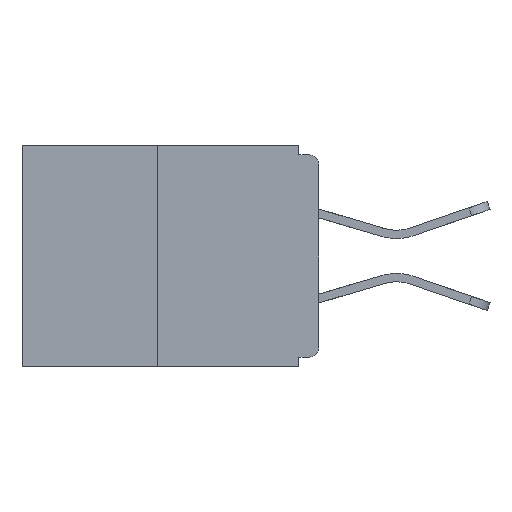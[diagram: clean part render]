
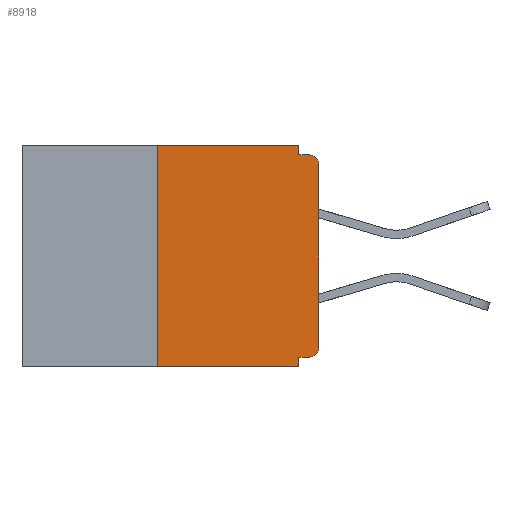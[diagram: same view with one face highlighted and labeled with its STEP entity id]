
A CAD part, left-side view. The second image highlights one B-rep face of the part: STEP entity #8918.
In plain terms, the highlighted planar face has unit normal (-1, 0, 0).
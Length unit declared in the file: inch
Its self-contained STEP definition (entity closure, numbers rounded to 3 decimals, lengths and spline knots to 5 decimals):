
#222 = EDGE_CURVE ( 'NONE', #14272, #4754, #8200, .T. ) ;
#387 = EDGE_CURVE ( 'NONE', #5098, #11218, #9555, .T. ) ;
#710 = DIRECTION ( 'NONE',  ( 0., -1., 0. ) ) ;
#914 = ORIENTED_EDGE ( 'NONE', *, *, #5044, .F. ) ;
#1134 = DIRECTION ( 'NONE',  ( 0., 0., -1. ) ) ;
#1265 = CARTESIAN_POINT ( 'NONE',  ( 0., 0.031, -0.015 ) ) ;
#1563 = CARTESIAN_POINT ( 'NONE',  ( 0., 0.031, -0.343 ) ) ;
#1713 = AXIS2_PLACEMENT_3D ( 'NONE', #7952, #4565, #1134 ) ;
#2033 = DIRECTION ( 'NONE',  ( 0., 0., -1. ) ) ;
#2289 = CARTESIAN_POINT ( 'NONE',  ( 0., 0.031, 0. ) ) ;
#2318 = ORIENTED_EDGE ( 'NONE', *, *, #8155, .F. ) ;
#2356 = AXIS2_PLACEMENT_3D ( 'NONE', #11083, #9074, #4626 ) ;
#2574 = CARTESIAN_POINT ( 'NONE',  ( 0., 0., -0.328 ) ) ;
#2588 = DIRECTION ( 'NONE',  ( 0., -1., 0. ) ) ;
#2750 = CARTESIAN_POINT ( 'NONE',  ( 0., 0.015, -0.313 ) ) ;
#2948 = VECTOR ( 'NONE', #13698, 39.37008 ) ;
#3143 = ORIENTED_EDGE ( 'NONE', *, *, #222, .T. ) ;
#3198 = EDGE_CURVE ( 'NONE', #12517, #14272, #5680, .T. ) ;
#3227 = VECTOR ( 'NONE', #10067, 39.37008 ) ;
#3420 = PLANE ( 'NONE',  #2356 ) ;
#3694 = EDGE_CURVE ( 'NONE', #13198, #4724, #12102, .T. ) ;
#3704 = CARTESIAN_POINT ( 'NONE',  ( 0., 0.015, -0.328 ) ) ;
#3873 = ORIENTED_EDGE ( 'NONE', *, *, #5990, .F. ) ;
#4414 = CARTESIAN_POINT ( 'NONE',  ( 0., 0.031, -0.343 ) ) ;
#4565 = DIRECTION ( 'NONE',  ( -1., 0., 0. ) ) ;
#4626 = DIRECTION ( 'NONE',  ( 0., 0., -1. ) ) ;
#4690 = ORIENTED_EDGE ( 'NONE', *, *, #10734, .T. ) ;
#4724 = VERTEX_POINT ( 'NONE', #1265 ) ;
#4754 = VERTEX_POINT ( 'NONE', #7933 ) ;
#5044 = EDGE_CURVE ( 'NONE', #11021, #13198, #8263, .T. ) ;
#5072 = VECTOR ( 'NONE', #11214, 39.37008 ) ;
#5098 = VERTEX_POINT ( 'NONE', #3704 ) ;
#5106 = VECTOR ( 'NONE', #2588, 39.37008 ) ;
#5109 = CARTESIAN_POINT ( 'NONE',  ( 0., 0., 0. ) ) ;
#5236 = CARTESIAN_POINT ( 'NONE',  ( 0., 0.25, 0. ) ) ;
#5571 = CARTESIAN_POINT ( 'NONE',  ( 0., 0., -0.313 ) ) ;
#5680 = LINE ( 'NONE', #5109, #7079 ) ;
#5990 = EDGE_CURVE ( 'NONE', #11218, #10954, #11665, .T. ) ;
#6112 = LINE ( 'NONE', #9053, #5072 ) ;
#6253 = CARTESIAN_POINT ( 'NONE',  ( 0., 0., -0.015 ) ) ;
#6674 = CARTESIAN_POINT ( 'NONE',  ( 0., 0.031, -0.328 ) ) ;
#6723 = ORIENTED_EDGE ( 'NONE', *, *, #13807, .F. ) ;
#6762 = CARTESIAN_POINT ( 'NONE',  ( 0., 0., -0.03 ) ) ;
#6983 = VECTOR ( 'NONE', #2033, 39.37008 ) ;
#7079 = VECTOR ( 'NONE', #9432, 39.37008 ) ;
#7489 = ORIENTED_EDGE ( 'NONE', *, *, #3198, .T. ) ;
#7549 = VERTEX_POINT ( 'NONE', #7600 ) ;
#7600 = CARTESIAN_POINT ( 'NONE',  ( 0., 0.25, -0.343 ) ) ;
#7933 = CARTESIAN_POINT ( 'NONE',  ( 0., 0.015, -0.015 ) ) ;
#7952 = CARTESIAN_POINT ( 'NONE',  ( 0., 0.015, -0.03 ) ) ;
#8155 = EDGE_CURVE ( 'NONE', #7549, #11021, #6112, .T. ) ;
#8200 = CIRCLE ( 'NONE', #1713, 0.015 ) ;
#8263 = LINE ( 'NONE', #11617, #5106 ) ;
#8517 = CIRCLE ( 'NONE', #13754, 0.015 ) ;
#8918 = ADVANCED_FACE ( 'NONE', ( #12882 ), #3420, .F. ) ;
#9046 = EDGE_CURVE ( 'NONE', #7549, #10954, #12865, .T. ) ;
#9053 = CARTESIAN_POINT ( 'NONE',  ( 0., 0.25, 0. ) ) ;
#9074 = DIRECTION ( 'NONE',  ( 1., 0., 0. ) ) ;
#9118 = CARTESIAN_POINT ( 'NONE',  ( 0., 0.46, -0.343 ) ) ;
#9313 = EDGE_LOOP ( 'NONE', ( #914, #2318, #13749, #3873, #13700, #4690, #7489, #3143, #6723, #13799 ) ) ;
#9432 = DIRECTION ( 'NONE',  ( 0., 0., 1. ) ) ;
#9473 = DIRECTION ( 'NONE',  ( 0., 0., -1. ) ) ;
#9555 = LINE ( 'NONE', #2574, #2948 ) ;
#9569 = DIRECTION ( 'NONE',  ( -1., 0., 0. ) ) ;
#10067 = DIRECTION ( 'NONE',  ( 0., 0., -1. ) ) ;
#10351 = LINE ( 'NONE', #6253, #12630 ) ;
#10734 = EDGE_CURVE ( 'NONE', #5098, #12517, #8517, .T. ) ;
#10954 = VERTEX_POINT ( 'NONE', #1563 ) ;
#11021 = VERTEX_POINT ( 'NONE', #5236 ) ;
#11083 = CARTESIAN_POINT ( 'NONE',  ( 0., 0.46, 0. ) ) ;
#11214 = DIRECTION ( 'NONE',  ( 0., 0., 1. ) ) ;
#11218 = VERTEX_POINT ( 'NONE', #6674 ) ;
#11617 = CARTESIAN_POINT ( 'NONE',  ( 0., 0.46, 0. ) ) ;
#11665 = LINE ( 'NONE', #4414, #6983 ) ;
#12102 = LINE ( 'NONE', #2289, #3227 ) ;
#12322 = CARTESIAN_POINT ( 'NONE',  ( 0., 0.031, 0. ) ) ;
#12461 = DIRECTION ( 'NONE',  ( 0., -1., 0. ) ) ;
#12517 = VERTEX_POINT ( 'NONE', #5571 ) ;
#12630 = VECTOR ( 'NONE', #710, 39.37008 ) ;
#12865 = LINE ( 'NONE', #9118, #13544 ) ;
#12882 = FACE_OUTER_BOUND ( 'NONE', #9313, .T. ) ;
#13198 = VERTEX_POINT ( 'NONE', #12322 ) ;
#13544 = VECTOR ( 'NONE', #12461, 39.37008 ) ;
#13698 = DIRECTION ( 'NONE',  ( 0., 1., 0. ) ) ;
#13700 = ORIENTED_EDGE ( 'NONE', *, *, #387, .F. ) ;
#13749 = ORIENTED_EDGE ( 'NONE', *, *, #9046, .T. ) ;
#13754 = AXIS2_PLACEMENT_3D ( 'NONE', #2750, #9569, #9473 ) ;
#13799 = ORIENTED_EDGE ( 'NONE', *, *, #3694, .F. ) ;
#13807 = EDGE_CURVE ( 'NONE', #4724, #4754, #10351, .T. ) ;
#14272 = VERTEX_POINT ( 'NONE', #6762 ) ;
